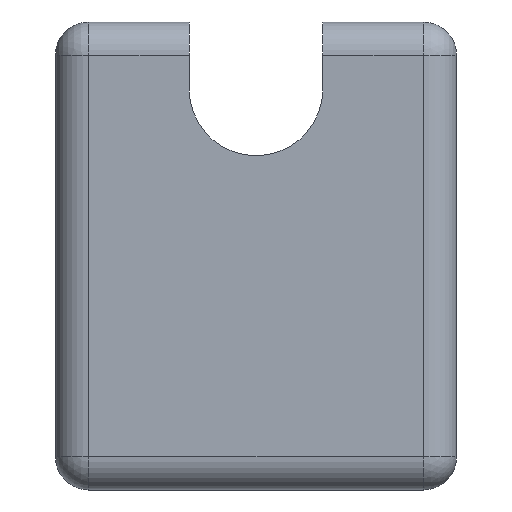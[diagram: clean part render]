
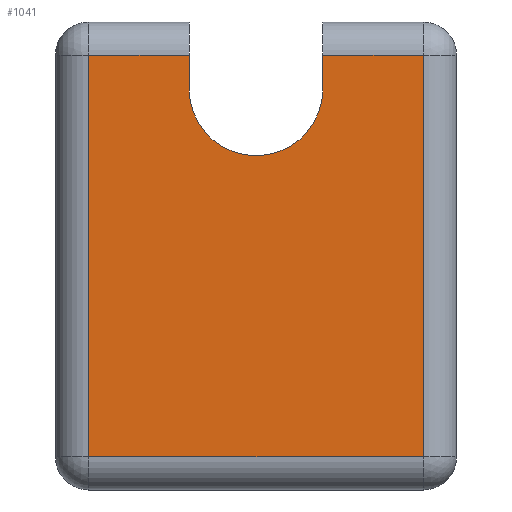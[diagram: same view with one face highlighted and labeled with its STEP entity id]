
A CAD part, left-side view. The second image highlights one B-rep face of the part: STEP entity #1041.
In plain terms, the highlighted planar face has unit normal (-1, 0, 0).
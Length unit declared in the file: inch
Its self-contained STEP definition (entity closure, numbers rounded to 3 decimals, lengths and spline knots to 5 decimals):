
#61 = EDGE_LOOP ( 'NONE', ( #1423, #2959, #456, #1615, #3440, #2545, #1887, #1014, #3390 ) ) ;
#225 = DIRECTION ( 'NONE',  ( 0., 1., 0. ) ) ;
#249 = FACE_OUTER_BOUND ( 'NONE', #61, .T. ) ;
#321 = DIRECTION ( 'NONE',  ( 0., 0., -1. ) ) ;
#393 = DIRECTION ( 'NONE',  ( 0., 0., 1. ) ) ;
#398 = VECTOR ( 'NONE', #4133, 39.37008 ) ;
#445 = VECTOR ( 'NONE', #321, 39.37008 ) ;
#456 = ORIENTED_EDGE ( 'NONE', *, *, #4175, .T. ) ;
#628 = CARTESIAN_POINT ( 'NONE',  ( 0., -0.3, 0.6 ) ) ;
#651 = LINE ( 'NONE', #2994, #2126 ) ;
#661 = VECTOR ( 'NONE', #1546, 39.37008 ) ;
#722 = VERTEX_POINT ( 'NONE', #3327 ) ;
#835 = CARTESIAN_POINT ( 'NONE',  ( 0., -0.4, 0.65 ) ) ;
#887 = DIRECTION ( 'NONE',  ( 0., 0., -1. ) ) ;
#930 = EDGE_CURVE ( 'NONE', #2786, #1882, #2601, .T. ) ;
#939 = CARTESIAN_POINT ( 'NONE',  ( 0., -0.4, 0.65 ) ) ;
#947 = EDGE_CURVE ( 'NONE', #1970, #1535, #2395, .T. ) ;
#1014 = ORIENTED_EDGE ( 'NONE', *, *, #2890, .T. ) ;
#1041 = ADVANCED_FACE ( 'NONE', ( #249 ), #2392, .F. ) ;
#1226 = VECTOR ( 'NONE', #887, 39.37008 ) ;
#1373 = CARTESIAN_POINT ( 'NONE',  ( 0., -0.05, 0.5 ) ) ;
#1378 = VECTOR ( 'NONE', #393, 39.37008 ) ;
#1423 = ORIENTED_EDGE ( 'NONE', *, *, #3149, .T. ) ;
#1428 = VERTEX_POINT ( 'NONE', #3412 ) ;
#1461 = AXIS2_PLACEMENT_3D ( 'NONE', #3848, #2883, #1913 ) ;
#1535 = VERTEX_POINT ( 'NONE', #3746 ) ;
#1546 = DIRECTION ( 'NONE',  ( 0., -1., 0. ) ) ;
#1615 = ORIENTED_EDGE ( 'NONE', *, *, #3568, .T. ) ;
#1621 = DIRECTION ( 'NONE',  ( 0., 1., 0. ) ) ;
#1657 = CARTESIAN_POINT ( 'NONE',  ( 0., -0.05, 0.65 ) ) ;
#1672 = CIRCLE ( 'NONE', #3236, 0.1 ) ;
#1679 = AXIS2_PLACEMENT_3D ( 'NONE', #4080, #3098, #2717 ) ;
#1882 = VERTEX_POINT ( 'NONE', #3583 ) ;
#1887 = ORIENTED_EDGE ( 'NONE', *, *, #2617, .T. ) ;
#1913 = DIRECTION ( 'NONE',  ( 0., 1., 0. ) ) ;
#1970 = VERTEX_POINT ( 'NONE', #3767 ) ;
#2126 = VECTOR ( 'NONE', #2360, 39.37008 ) ;
#2337 = CARTESIAN_POINT ( 'NONE',  ( 0., -0.3, 0.5 ) ) ;
#2360 = DIRECTION ( 'NONE',  ( 0., 0., -1. ) ) ;
#2392 = PLANE ( 'NONE',  #1679 ) ;
#2395 = LINE ( 'NONE', #2833, #661 ) ;
#2545 = ORIENTED_EDGE ( 'NONE', *, *, #930, .F. ) ;
#2601 = LINE ( 'NONE', #3516, #1226 ) ;
#2617 = EDGE_CURVE ( 'NONE', #2786, #4011, #3300, .T. ) ;
#2686 = VECTOR ( 'NONE', #225, 39.37008 ) ;
#2717 = DIRECTION ( 'NONE',  ( 0., 1., 0. ) ) ;
#2786 = VERTEX_POINT ( 'NONE', #4158 ) ;
#2811 = EDGE_CURVE ( 'NONE', #2941, #1882, #3102, .T. ) ;
#2833 = CARTESIAN_POINT ( 'NONE',  ( 0., 0., 0.05 ) ) ;
#2883 = DIRECTION ( 'NONE',  ( 1., 0., 0. ) ) ;
#2890 = EDGE_CURVE ( 'NONE', #4011, #1970, #2902, .T. ) ;
#2902 = LINE ( 'NONE', #1373, #445 ) ;
#2941 = VERTEX_POINT ( 'NONE', #2337 ) ;
#2959 = ORIENTED_EDGE ( 'NONE', *, *, #3500, .T. ) ;
#2994 = CARTESIAN_POINT ( 'NONE',  ( 0., -0.4, 0.7 ) ) ;
#3098 = DIRECTION ( 'NONE',  ( 1., 0., 0. ) ) ;
#3102 = CIRCLE ( 'NONE', #1461, 0.1 ) ;
#3149 = EDGE_CURVE ( 'NONE', #1535, #722, #3206, .T. ) ;
#3179 = CARTESIAN_POINT ( 'NONE',  ( 0., -0.05, 0.65 ) ) ;
#3206 = LINE ( 'NONE', #3984, #1378 ) ;
#3236 = AXIS2_PLACEMENT_3D ( 'NONE', #628, #3578, #1621 ) ;
#3300 = LINE ( 'NONE', #3179, #398 ) ;
#3327 = CARTESIAN_POINT ( 'NONE',  ( 0., -0.55, 0.65 ) ) ;
#3390 = ORIENTED_EDGE ( 'NONE', *, *, #947, .T. ) ;
#3412 = CARTESIAN_POINT ( 'NONE',  ( 0., -0.4, 0.6 ) ) ;
#3440 = ORIENTED_EDGE ( 'NONE', *, *, #2811, .T. ) ;
#3500 = EDGE_CURVE ( 'NONE', #722, #3850, #3601, .T. ) ;
#3516 = CARTESIAN_POINT ( 'NONE',  ( 0., -0.2, 0.7 ) ) ;
#3568 = EDGE_CURVE ( 'NONE', #1428, #2941, #1672, .T. ) ;
#3578 = DIRECTION ( 'NONE',  ( 1., 0., 0. ) ) ;
#3583 = CARTESIAN_POINT ( 'NONE',  ( 0., -0.2, 0.6 ) ) ;
#3601 = LINE ( 'NONE', #939, #2686 ) ;
#3746 = CARTESIAN_POINT ( 'NONE',  ( 0., -0.55, 0.05 ) ) ;
#3767 = CARTESIAN_POINT ( 'NONE',  ( 0., -0.05, 0.05 ) ) ;
#3848 = CARTESIAN_POINT ( 'NONE',  ( 0., -0.3, 0.6 ) ) ;
#3850 = VERTEX_POINT ( 'NONE', #835 ) ;
#3984 = CARTESIAN_POINT ( 'NONE',  ( 0., -0.55, 0.5 ) ) ;
#4011 = VERTEX_POINT ( 'NONE', #1657 ) ;
#4080 = CARTESIAN_POINT ( 'NONE',  ( 0., 0., 0.5 ) ) ;
#4133 = DIRECTION ( 'NONE',  ( 0., 1., 0. ) ) ;
#4158 = CARTESIAN_POINT ( 'NONE',  ( 0., -0.2, 0.65 ) ) ;
#4175 = EDGE_CURVE ( 'NONE', #3850, #1428, #651, .T. ) ;
